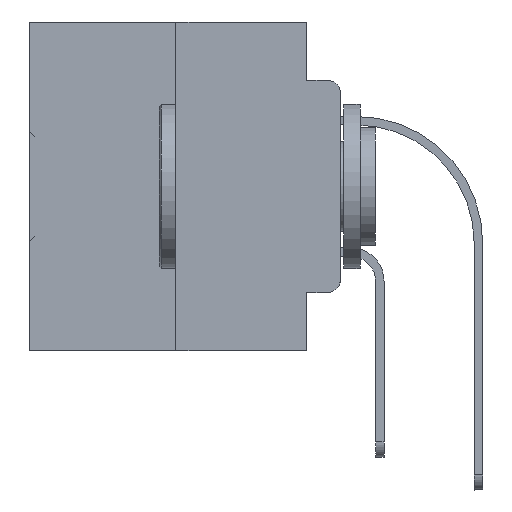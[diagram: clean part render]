
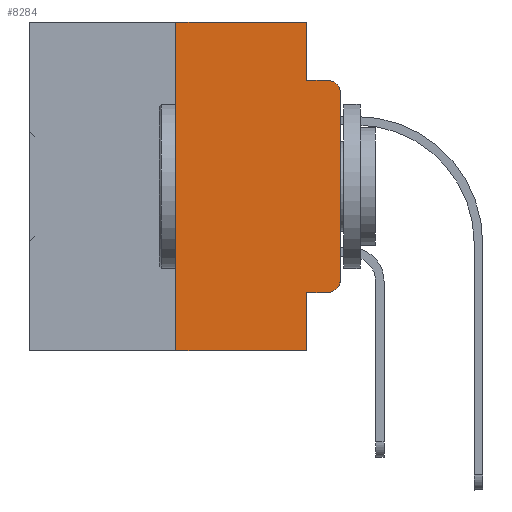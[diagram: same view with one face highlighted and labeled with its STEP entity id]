
A CAD part, left-side view. The second image highlights one B-rep face of the part: STEP entity #8284.
In plain terms, the highlighted planar face has unit normal (-1, 0, 0).
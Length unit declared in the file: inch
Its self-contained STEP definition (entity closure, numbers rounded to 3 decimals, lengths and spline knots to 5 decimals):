
#12 = LINE ( 'NONE', #5978, #32886 ) ;
#39 = VERTEX_POINT ( 'NONE', #30893 ) ;
#210 = DIRECTION ( 'NONE',  ( 0., -1., 0. ) ) ;
#903 = VERTEX_POINT ( 'NONE', #26274 ) ;
#1041 = VECTOR ( 'NONE', #210, 39.37008 ) ;
#1136 = CARTESIAN_POINT ( 'NONE',  ( 0., 0.051, -0.4115 ) ) ;
#1554 = CARTESIAN_POINT ( 'NONE',  ( 0., 0., -0.1085 ) ) ;
#1772 = CARTESIAN_POINT ( 'NONE',  ( 0., 0.02, -0.4115 ) ) ;
#2000 = VERTEX_POINT ( 'NONE', #32953 ) ;
#2729 = VERTEX_POINT ( 'NONE', #36578 ) ;
#3388 = CARTESIAN_POINT ( 'NONE',  ( 0., 0.473, 0. ) ) ;
#4695 = DIRECTION ( 'NONE',  ( 0., -1., 0. ) ) ;
#5548 = EDGE_CURVE ( 'NONE', #30347, #2000, #38207, .T. ) ;
#5978 = CARTESIAN_POINT ( 'NONE',  ( 0., 0.051, 0. ) ) ;
#6282 = DIRECTION ( 'NONE',  ( 0., 0., 1. ) ) ;
#6329 = EDGE_CURVE ( 'NONE', #2729, #903, #22535, .T. ) ;
#7014 = DIRECTION ( 'NONE',  ( 1., 0., 0. ) ) ;
#7409 = VERTEX_POINT ( 'NONE', #9505 ) ;
#8038 = DIRECTION ( 'NONE',  ( 0., 0., -1. ) ) ;
#8152 = CARTESIAN_POINT ( 'NONE',  ( 0., 0.051, 0. ) ) ;
#8284 = ADVANCED_FACE ( 'NONE', ( #35704 ), #8633, .F. ) ;
#8633 = PLANE ( 'NONE',  #25083 ) ;
#8732 = EDGE_CURVE ( 'NONE', #22376, #38073, #21810, .T. ) ;
#8735 = CIRCLE ( 'NONE', #13782, 0.02 ) ;
#8868 = VERTEX_POINT ( 'NONE', #1772 ) ;
#9326 = EDGE_CURVE ( 'NONE', #26875, #903, #8735, .T. ) ;
#9505 = CARTESIAN_POINT ( 'NONE',  ( 0., 0., -0.3915 ) ) ;
#10627 = CARTESIAN_POINT ( 'NONE',  ( 0., 0.02, -0.1085 ) ) ;
#10680 = LINE ( 'NONE', #35197, #36065 ) ;
#10976 = VECTOR ( 'NONE', #24528, 39.37008 ) ;
#11213 = DIRECTION ( 'NONE',  ( -1., 0., 0. ) ) ;
#13782 = AXIS2_PLACEMENT_3D ( 'NONE', #10627, #11213, #32357 ) ;
#14456 = DIRECTION ( 'NONE',  ( 0., -1., 0. ) ) ;
#15764 = CARTESIAN_POINT ( 'NONE',  ( 0., 0.25, -0.5 ) ) ;
#16958 = ORIENTED_EDGE ( 'NONE', *, *, #23441, .F. ) ;
#16988 = CIRCLE ( 'NONE', #20151, 0.02 ) ;
#17311 = VECTOR ( 'NONE', #4695, 39.37008 ) ;
#17984 = ORIENTED_EDGE ( 'NONE', *, *, #8732, .F. ) ;
#19049 = EDGE_CURVE ( 'NONE', #7409, #26875, #22114, .T. ) ;
#19698 = CARTESIAN_POINT ( 'NONE',  ( 0., 0.051, 0. ) ) ;
#20151 = AXIS2_PLACEMENT_3D ( 'NONE', #20487, #31958, #8038 ) ;
#20194 = ORIENTED_EDGE ( 'NONE', *, *, #6329, .F. ) ;
#20487 = CARTESIAN_POINT ( 'NONE',  ( 0., 0.02, -0.3915 ) ) ;
#20700 = CARTESIAN_POINT ( 'NONE',  ( 0., 0.473, 0. ) ) ;
#21636 = EDGE_CURVE ( 'NONE', #38073, #2729, #35236, .T. ) ;
#21810 = LINE ( 'NONE', #3388, #1041 ) ;
#22054 = DIRECTION ( 'NONE',  ( 0., 0., -1. ) ) ;
#22114 = LINE ( 'NONE', #30809, #23804 ) ;
#22302 = ORIENTED_EDGE ( 'NONE', *, *, #29341, .F. ) ;
#22376 = VERTEX_POINT ( 'NONE', #26585 ) ;
#22535 = LINE ( 'NONE', #25478, #17311 ) ;
#22777 = ORIENTED_EDGE ( 'NONE', *, *, #19049, .T. ) ;
#22915 = ORIENTED_EDGE ( 'NONE', *, *, #9326, .T. ) ;
#23441 = EDGE_CURVE ( 'NONE', #30347, #22376, #10680, .T. ) ;
#23509 = ORIENTED_EDGE ( 'NONE', *, *, #26292, .T. ) ;
#23804 = VECTOR ( 'NONE', #6282, 39.37008 ) ;
#24528 = DIRECTION ( 'NONE',  ( 0., -1., 0. ) ) ;
#25083 = AXIS2_PLACEMENT_3D ( 'NONE', #20700, #7014, #22054 ) ;
#25478 = CARTESIAN_POINT ( 'NONE',  ( 0., 0.051, -0.0885 ) ) ;
#25515 = DIRECTION ( 'NONE',  ( 0., 0., 1. ) ) ;
#26136 = VECTOR ( 'NONE', #14456, 39.37008 ) ;
#26274 = CARTESIAN_POINT ( 'NONE',  ( 0., 0.02, -0.0885 ) ) ;
#26292 = EDGE_CURVE ( 'NONE', #39, #8868, #34182, .T. ) ;
#26585 = CARTESIAN_POINT ( 'NONE',  ( 0., 0.25, 0. ) ) ;
#26875 = VERTEX_POINT ( 'NONE', #1554 ) ;
#27417 = EDGE_CURVE ( 'NONE', #8868, #7409, #16988, .T. ) ;
#29341 = EDGE_CURVE ( 'NONE', #39, #2000, #12, .T. ) ;
#29499 = CARTESIAN_POINT ( 'NONE',  ( 0., 0.473, -0.5 ) ) ;
#29727 = VECTOR ( 'NONE', #35432, 39.37008 ) ;
#30123 = DIRECTION ( 'NONE',  ( 0., 0., -1. ) ) ;
#30347 = VERTEX_POINT ( 'NONE', #15764 ) ;
#30588 = ORIENTED_EDGE ( 'NONE', *, *, #27417, .T. ) ;
#30809 = CARTESIAN_POINT ( 'NONE',  ( 0., 0., 0. ) ) ;
#30893 = CARTESIAN_POINT ( 'NONE',  ( 0., 0.051, -0.4115 ) ) ;
#31905 = ORIENTED_EDGE ( 'NONE', *, *, #21636, .F. ) ;
#31958 = DIRECTION ( 'NONE',  ( -1., 0., 0. ) ) ;
#32357 = DIRECTION ( 'NONE',  ( 0., 0., -1. ) ) ;
#32786 = ORIENTED_EDGE ( 'NONE', *, *, #5548, .T. ) ;
#32886 = VECTOR ( 'NONE', #30123, 39.37008 ) ;
#32953 = CARTESIAN_POINT ( 'NONE',  ( 0., 0.051, -0.5 ) ) ;
#34182 = LINE ( 'NONE', #1136, #10976 ) ;
#35197 = CARTESIAN_POINT ( 'NONE',  ( 0., 0.25, 0. ) ) ;
#35236 = LINE ( 'NONE', #8152, #29727 ) ;
#35432 = DIRECTION ( 'NONE',  ( 0., 0., -1. ) ) ;
#35704 = FACE_OUTER_BOUND ( 'NONE', #38540, .T. ) ;
#36065 = VECTOR ( 'NONE', #25515, 39.37008 ) ;
#36578 = CARTESIAN_POINT ( 'NONE',  ( 0., 0.051, -0.0885 ) ) ;
#38073 = VERTEX_POINT ( 'NONE', #19698 ) ;
#38207 = LINE ( 'NONE', #29499, #26136 ) ;
#38540 = EDGE_LOOP ( 'NONE', ( #22777, #22915, #20194, #31905, #17984, #16958, #32786, #22302, #23509, #30588 ) ) ;
